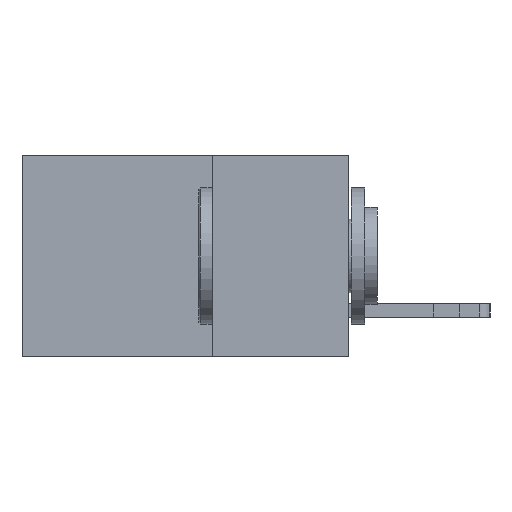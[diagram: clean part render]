
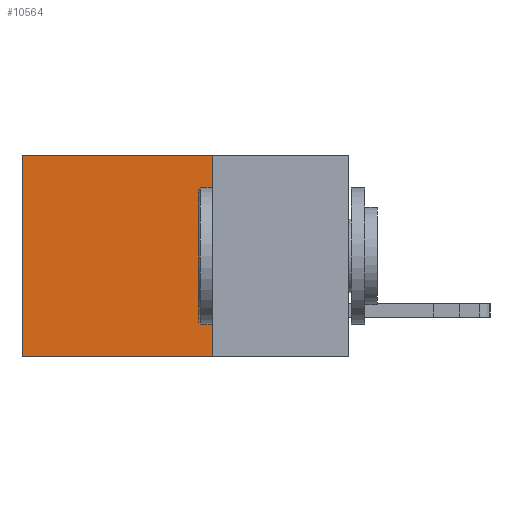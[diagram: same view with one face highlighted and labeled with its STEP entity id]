
A CAD part, left-side view. The second image highlights one B-rep face of the part: STEP entity #10564.
In plain terms, the highlighted planar face has unit normal (-1, 0, 0).
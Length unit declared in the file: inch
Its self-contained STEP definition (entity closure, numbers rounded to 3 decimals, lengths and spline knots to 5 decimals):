
#362 = EDGE_CURVE ( 'NONE', #9232, #10159, #6344, .T. ) ;
#437 = ORIENTED_EDGE ( 'NONE', *, *, #7738, .T. ) ;
#651 = LINE ( 'NONE', #9483, #8063 ) ;
#958 = DIRECTION ( 'NONE',  ( 0., 0., -1. ) ) ;
#1182 = LINE ( 'NONE', #6723, #3336 ) ;
#1234 = PLANE ( 'NONE',  #4101 ) ;
#1277 = VECTOR ( 'NONE', #958, 39.37008 ) ;
#1400 = ORIENTED_EDGE ( 'NONE', *, *, #362, .F. ) ;
#1814 = EDGE_CURVE ( 'NONE', #10159, #9214, #1182, .T. ) ;
#2825 = EDGE_LOOP ( 'NONE', ( #437, #6366, #1400, #3595 ) ) ;
#3082 = DIRECTION ( 'NONE',  ( 0., 0., -1. ) ) ;
#3336 = VECTOR ( 'NONE', #9997, 39.37008 ) ;
#3488 = DIRECTION ( 'NONE',  ( 0., 1., 0. ) ) ;
#3595 = ORIENTED_EDGE ( 'NONE', *, *, #8208, .T. ) ;
#3949 = VECTOR ( 'NONE', #5194, 39.37008 ) ;
#4101 = AXIS2_PLACEMENT_3D ( 'NONE', #7500, #8318, #3082 ) ;
#4935 = CARTESIAN_POINT ( 'NONE',  ( 0.2615, 0.6, -0.37 ) ) ;
#5194 = DIRECTION ( 'NONE',  ( 0., 0., -1. ) ) ;
#5853 = CARTESIAN_POINT ( 'NONE',  ( 0.2615, 0.6, 0. ) ) ;
#6344 = LINE ( 'NONE', #10561, #3949 ) ;
#6366 = ORIENTED_EDGE ( 'NONE', *, *, #1814, .F. ) ;
#6391 = CARTESIAN_POINT ( 'NONE',  ( 0.2615, 0.6, -0.37 ) ) ;
#6649 = VERTEX_POINT ( 'NONE', #5853 ) ;
#6723 = CARTESIAN_POINT ( 'NONE',  ( 0.2615, 0.25, -0.37 ) ) ;
#7500 = CARTESIAN_POINT ( 'NONE',  ( 0.2615, 0.25, -0.37 ) ) ;
#7738 = EDGE_CURVE ( 'NONE', #6649, #9214, #8333, .T. ) ;
#7784 = CARTESIAN_POINT ( 'NONE',  ( 0.2615, 0.25, -0.37 ) ) ;
#8063 = VECTOR ( 'NONE', #3488, 39.37008 ) ;
#8208 = EDGE_CURVE ( 'NONE', #9232, #6649, #651, .T. ) ;
#8318 = DIRECTION ( 'NONE',  ( 1., 0., 0. ) ) ;
#8333 = LINE ( 'NONE', #6391, #1277 ) ;
#9186 = CARTESIAN_POINT ( 'NONE',  ( 0.2615, 0.25, 0. ) ) ;
#9214 = VERTEX_POINT ( 'NONE', #4935 ) ;
#9232 = VERTEX_POINT ( 'NONE', #9186 ) ;
#9483 = CARTESIAN_POINT ( 'NONE',  ( 0.2615, 0.25, 0. ) ) ;
#9997 = DIRECTION ( 'NONE',  ( 0., 1., 0. ) ) ;
#10159 = VERTEX_POINT ( 'NONE', #7784 ) ;
#10428 = FACE_OUTER_BOUND ( 'NONE', #2825, .T. ) ;
#10561 = CARTESIAN_POINT ( 'NONE',  ( 0.2615, 0.25, -0.37 ) ) ;
#10564 = ADVANCED_FACE ( 'NONE', ( #10428 ), #1234, .F. ) ;
